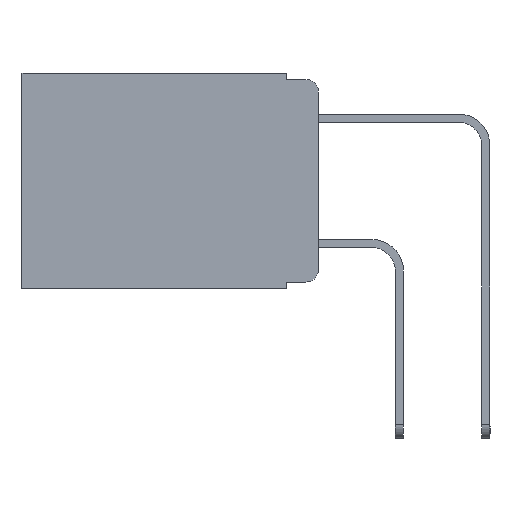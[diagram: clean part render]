
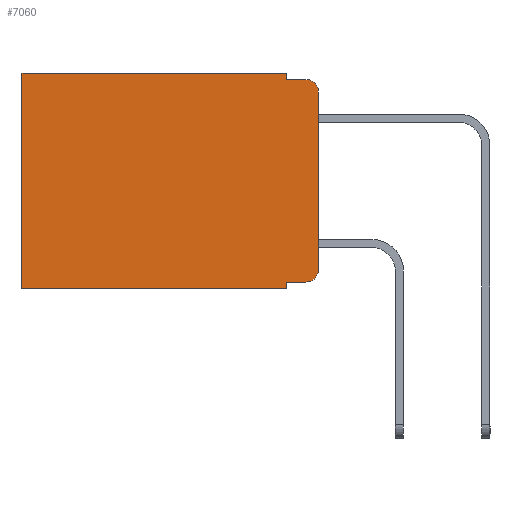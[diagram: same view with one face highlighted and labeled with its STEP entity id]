
A CAD part, left-side view. The second image highlights one B-rep face of the part: STEP entity #7060.
In plain terms, the highlighted planar face has unit normal (-1, 0, 0).
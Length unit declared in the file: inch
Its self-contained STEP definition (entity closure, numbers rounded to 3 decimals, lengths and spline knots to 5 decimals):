
#28 = DIRECTION ( 'NONE',  ( 0., 0., -1. ) ) ;
#476 = VECTOR ( 'NONE', #3531, 39.37008 ) ;
#673 = DIRECTION ( 'NONE',  ( 0., 0., -1. ) ) ;
#776 = VECTOR ( 'NONE', #2281, 39.37008 ) ;
#863 = EDGE_CURVE ( 'NONE', #8828, #7139, #3003, .T. ) ;
#959 = ORIENTED_EDGE ( 'NONE', *, *, #7884, .F. ) ;
#1027 = LINE ( 'NONE', #2415, #11495 ) ;
#1199 = VERTEX_POINT ( 'NONE', #6611 ) ;
#1540 = AXIS2_PLACEMENT_3D ( 'NONE', #4032, #9125, #28 ) ;
#1628 = CARTESIAN_POINT ( 'NONE',  ( 0.298, 0.02, -0.01 ) ) ;
#2266 = EDGE_CURVE ( 'NONE', #6050, #8828, #4397, .T. ) ;
#2281 = DIRECTION ( 'NONE',  ( 0., 0., -1. ) ) ;
#2345 = CARTESIAN_POINT ( 'NONE',  ( 0.298, 0.051, 0. ) ) ;
#2415 = CARTESIAN_POINT ( 'NONE',  ( 0.298, 0., 0. ) ) ;
#2536 = VECTOR ( 'NONE', #673, 39.37008 ) ;
#2687 = VERTEX_POINT ( 'NONE', #7525 ) ;
#3003 = LINE ( 'NONE', #11249, #7146 ) ;
#3176 = CARTESIAN_POINT ( 'NONE',  ( 0.298, 0.473, -0.343 ) ) ;
#3236 = VERTEX_POINT ( 'NONE', #1628 ) ;
#3331 = VERTEX_POINT ( 'NONE', #11001 ) ;
#3516 = ORIENTED_EDGE ( 'NONE', *, *, #9439, .T. ) ;
#3531 = DIRECTION ( 'NONE',  ( 0., 0., -1. ) ) ;
#3838 = DIRECTION ( 'NONE',  ( 0., -1., 0. ) ) ;
#3872 = CARTESIAN_POINT ( 'NONE',  ( 0.298, 0.02, -0.313 ) ) ;
#4032 = CARTESIAN_POINT ( 'NONE',  ( 0.298, 0., 0. ) ) ;
#4103 = PLANE ( 'NONE',  #1540 ) ;
#4397 = LINE ( 'NONE', #2345, #776 ) ;
#4454 = CARTESIAN_POINT ( 'NONE',  ( 0.298, 0.02, -0.03 ) ) ;
#4521 = AXIS2_PLACEMENT_3D ( 'NONE', #4454, #11703, #10562 ) ;
#4534 = ORIENTED_EDGE ( 'NONE', *, *, #9409, .T. ) ;
#4575 = VECTOR ( 'NONE', #5349, 39.37008 ) ;
#4846 = CARTESIAN_POINT ( 'NONE',  ( 0.298, 0.051, -0.01 ) ) ;
#4939 = DIRECTION ( 'NONE',  ( 0., 1., 0. ) ) ;
#5038 = FACE_OUTER_BOUND ( 'NONE', #5147, .T. ) ;
#5147 = EDGE_LOOP ( 'NONE', ( #9145, #11321, #11697, #959, #7747, #3516, #7538, #5470, #4534, #6249 ) ) ;
#5349 = DIRECTION ( 'NONE',  ( 0., -1., 0. ) ) ;
#5470 = ORIENTED_EDGE ( 'NONE', *, *, #2266, .F. ) ;
#5908 = EDGE_CURVE ( 'NONE', #11029, #3236, #11176, .T. ) ;
#6050 = VERTEX_POINT ( 'NONE', #7669 ) ;
#6072 = CARTESIAN_POINT ( 'NONE',  ( 0.298, 0., -0.03 ) ) ;
#6123 = LINE ( 'NONE', #4846, #10568 ) ;
#6249 = ORIENTED_EDGE ( 'NONE', *, *, #6502, .T. ) ;
#6481 = LINE ( 'NONE', #7485, #12081 ) ;
#6502 = EDGE_CURVE ( 'NONE', #11236, #1199, #8569, .T. ) ;
#6611 = CARTESIAN_POINT ( 'NONE',  ( 0.298, 0., -0.313 ) ) ;
#7060 = ADVANCED_FACE ( 'NONE', ( #5038 ), #4103, .F. ) ;
#7139 = VERTEX_POINT ( 'NONE', #3176 ) ;
#7146 = VECTOR ( 'NONE', #4939, 39.37008 ) ;
#7485 = CARTESIAN_POINT ( 'NONE',  ( 0.298, 0.473, 0. ) ) ;
#7525 = CARTESIAN_POINT ( 'NONE',  ( 0.298, 0.473, 0. ) ) ;
#7538 = ORIENTED_EDGE ( 'NONE', *, *, #863, .F. ) ;
#7669 = CARTESIAN_POINT ( 'NONE',  ( 0.298, 0.051, -0.333 ) ) ;
#7747 = ORIENTED_EDGE ( 'NONE', *, *, #10849, .T. ) ;
#7884 = EDGE_CURVE ( 'NONE', #9142, #3331, #12737, .T. ) ;
#8569 = CIRCLE ( 'NONE', #11371, 0.02 ) ;
#8828 = VERTEX_POINT ( 'NONE', #12421 ) ;
#8843 = DIRECTION ( 'NONE',  ( -1., 0., 0. ) ) ;
#9038 = DIRECTION ( 'NONE',  ( 0., 0., -1. ) ) ;
#9125 = DIRECTION ( 'NONE',  ( 1., 0., 0. ) ) ;
#9142 = VERTEX_POINT ( 'NONE', #12877 ) ;
#9145 = ORIENTED_EDGE ( 'NONE', *, *, #13019, .F. ) ;
#9259 = DIRECTION ( 'NONE',  ( 0., 1., 0. ) ) ;
#9409 = EDGE_CURVE ( 'NONE', #6050, #11236, #10454, .T. ) ;
#9439 = EDGE_CURVE ( 'NONE', #2687, #7139, #6481, .T. ) ;
#9692 = LINE ( 'NONE', #12933, #476 ) ;
#10224 = EDGE_CURVE ( 'NONE', #3331, #3236, #6123, .T. ) ;
#10454 = LINE ( 'NONE', #12532, #4575 ) ;
#10471 = CARTESIAN_POINT ( 'NONE',  ( 0.298, 0.02, -0.333 ) ) ;
#10562 = DIRECTION ( 'NONE',  ( 0., 0., -1. ) ) ;
#10568 = VECTOR ( 'NONE', #3838, 39.37008 ) ;
#10574 = DIRECTION ( 'NONE',  ( 0., 0., -1. ) ) ;
#10849 = EDGE_CURVE ( 'NONE', #9142, #2687, #1027, .T. ) ;
#10920 = CARTESIAN_POINT ( 'NONE',  ( 0.298, 0.051, 0. ) ) ;
#11001 = CARTESIAN_POINT ( 'NONE',  ( 0.298, 0.051, -0.01 ) ) ;
#11029 = VERTEX_POINT ( 'NONE', #6072 ) ;
#11176 = CIRCLE ( 'NONE', #4521, 0.02 ) ;
#11236 = VERTEX_POINT ( 'NONE', #10471 ) ;
#11249 = CARTESIAN_POINT ( 'NONE',  ( 0.298, 0., -0.343 ) ) ;
#11321 = ORIENTED_EDGE ( 'NONE', *, *, #5908, .T. ) ;
#11371 = AXIS2_PLACEMENT_3D ( 'NONE', #3872, #8843, #9038 ) ;
#11495 = VECTOR ( 'NONE', #9259, 39.37008 ) ;
#11697 = ORIENTED_EDGE ( 'NONE', *, *, #10224, .F. ) ;
#11703 = DIRECTION ( 'NONE',  ( -1., 0., 0. ) ) ;
#12081 = VECTOR ( 'NONE', #10574, 39.37008 ) ;
#12421 = CARTESIAN_POINT ( 'NONE',  ( 0.298, 0.051, -0.343 ) ) ;
#12532 = CARTESIAN_POINT ( 'NONE',  ( 0.298, 0.051, -0.333 ) ) ;
#12737 = LINE ( 'NONE', #10920, #2536 ) ;
#12877 = CARTESIAN_POINT ( 'NONE',  ( 0.298, 0.051, 0. ) ) ;
#12933 = CARTESIAN_POINT ( 'NONE',  ( 0.298, 0., 0. ) ) ;
#13019 = EDGE_CURVE ( 'NONE', #11029, #1199, #9692, .T. ) ;
